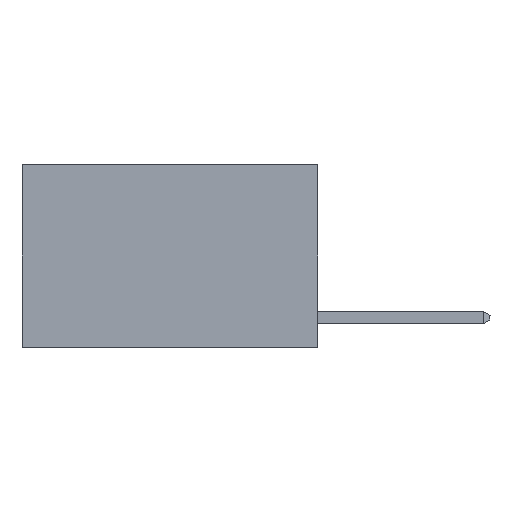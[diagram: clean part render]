
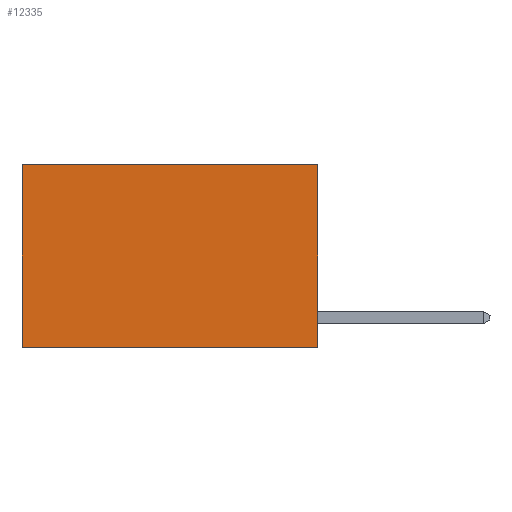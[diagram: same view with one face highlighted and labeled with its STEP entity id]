
A CAD part, left-side view. The second image highlights one B-rep face of the part: STEP entity #12335.
In plain terms, the highlighted planar face has unit normal (-1, 0, 0).
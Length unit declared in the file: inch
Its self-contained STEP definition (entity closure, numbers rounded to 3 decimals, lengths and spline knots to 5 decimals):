
#707 = CARTESIAN_POINT ( 'NONE',  ( 0.2625, 0., 0. ) ) ;
#2071 = FACE_OUTER_BOUND ( 'NONE', #3665, .T. ) ;
#2147 = DIRECTION ( 'NONE',  ( 0., 0., -1. ) ) ;
#2259 = DIRECTION ( 'NONE',  ( 0., 1., 0. ) ) ;
#2384 = ORIENTED_EDGE ( 'NONE', *, *, #5718, .F. ) ;
#2515 = VECTOR ( 'NONE', #8727, 39.37008 ) ;
#3198 = CARTESIAN_POINT ( 'NONE',  ( 0.2625, 0., 0. ) ) ;
#3213 = ORIENTED_EDGE ( 'NONE', *, *, #9078, .T. ) ;
#3565 = AXIS2_PLACEMENT_3D ( 'NONE', #3198, #11263, #4477 ) ;
#3665 = EDGE_LOOP ( 'NONE', ( #5191, #2384, #13165, #3213 ) ) ;
#3909 = DIRECTION ( 'NONE',  ( 0., 1., 0. ) ) ;
#4477 = DIRECTION ( 'NONE',  ( 0., 0., -1. ) ) ;
#4723 = VERTEX_POINT ( 'NONE', #14033 ) ;
#5191 = ORIENTED_EDGE ( 'NONE', *, *, #5511, .T. ) ;
#5223 = VERTEX_POINT ( 'NONE', #7587 ) ;
#5312 = VECTOR ( 'NONE', #2259, 39.37008 ) ;
#5511 = EDGE_CURVE ( 'NONE', #9760, #5223, #16602, .T. ) ;
#5718 = EDGE_CURVE ( 'NONE', #4723, #5223, #7252, .T. ) ;
#6054 = CARTESIAN_POINT ( 'NONE',  ( 0.2625, 0., 0. ) ) ;
#6062 = PLANE ( 'NONE',  #3565 ) ;
#6233 = CARTESIAN_POINT ( 'NONE',  ( 0.2625, 0., -0.37 ) ) ;
#7252 = LINE ( 'NONE', #6233, #5312 ) ;
#7587 = CARTESIAN_POINT ( 'NONE',  ( 0.2625, 0.6, -0.37 ) ) ;
#8715 = CARTESIAN_POINT ( 'NONE',  ( 0.2625, 0.6, 0. ) ) ;
#8727 = DIRECTION ( 'NONE',  ( 0., 0., -1. ) ) ;
#9078 = EDGE_CURVE ( 'NONE', #14862, #9760, #13444, .T. ) ;
#9760 = VERTEX_POINT ( 'NONE', #8715 ) ;
#9799 = VECTOR ( 'NONE', #2147, 39.37008 ) ;
#10741 = EDGE_CURVE ( 'NONE', #14862, #4723, #11522, .T. ) ;
#11263 = DIRECTION ( 'NONE',  ( 1., 0., 0. ) ) ;
#11422 = VECTOR ( 'NONE', #3909, 39.37008 ) ;
#11522 = LINE ( 'NONE', #6054, #9799 ) ;
#12335 = ADVANCED_FACE ( 'NONE', ( #2071 ), #6062, .F. ) ;
#13153 = CARTESIAN_POINT ( 'NONE',  ( 0.2625, 0., 0. ) ) ;
#13165 = ORIENTED_EDGE ( 'NONE', *, *, #10741, .F. ) ;
#13444 = LINE ( 'NONE', #13153, #11422 ) ;
#13948 = CARTESIAN_POINT ( 'NONE',  ( 0.2625, 0.6, 0. ) ) ;
#14033 = CARTESIAN_POINT ( 'NONE',  ( 0.2625, 0., -0.37 ) ) ;
#14862 = VERTEX_POINT ( 'NONE', #707 ) ;
#16602 = LINE ( 'NONE', #13948, #2515 ) ;
